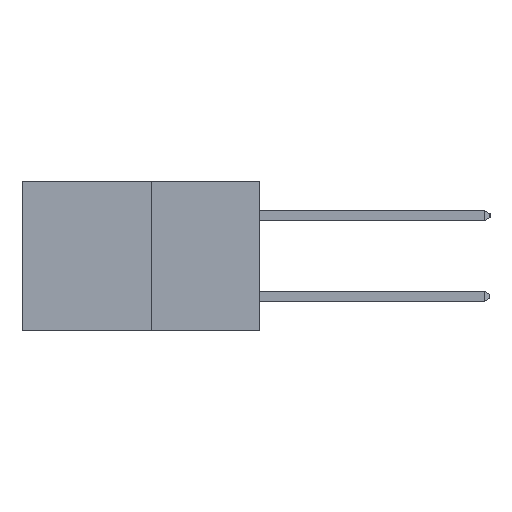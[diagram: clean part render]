
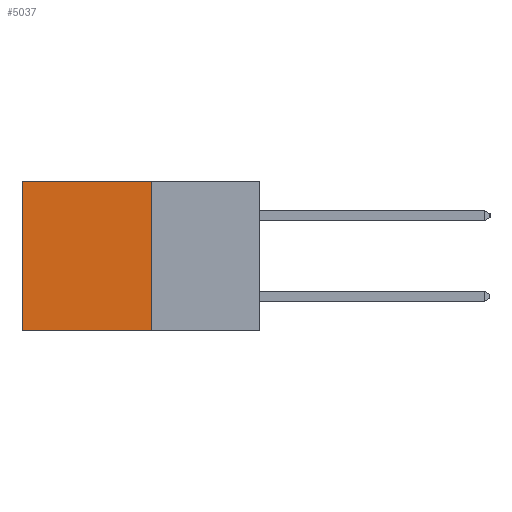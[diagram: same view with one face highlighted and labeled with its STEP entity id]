
A CAD part, left-side view. The second image highlights one B-rep face of the part: STEP entity #5037.
In plain terms, the highlighted planar face has unit normal (-1, 0, 0).
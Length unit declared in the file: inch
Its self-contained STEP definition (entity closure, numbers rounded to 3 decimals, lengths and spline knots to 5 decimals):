
#45 = CARTESIAN_POINT ( 'NONE',  ( 0.277, 0.59, -0.37 ) ) ;
#147 = CARTESIAN_POINT ( 'NONE',  ( 0.277, 0.27, 0. ) ) ;
#843 = VECTOR ( 'NONE', #1164, 39.37008 ) ;
#1095 = LINE ( 'NONE', #45, #843 ) ;
#1164 = DIRECTION ( 'NONE',  ( 0., 0., -1. ) ) ;
#1592 = LINE ( 'NONE', #4314, #1824 ) ;
#1748 = VECTOR ( 'NONE', #6209, 39.37008 ) ;
#1824 = VECTOR ( 'NONE', #4326, 39.37008 ) ;
#2028 = CARTESIAN_POINT ( 'NONE',  ( 0.277, 0.59, -0.37 ) ) ;
#2149 = VERTEX_POINT ( 'NONE', #147 ) ;
#2707 = VECTOR ( 'NONE', #7558, 39.37008 ) ;
#2893 = VERTEX_POINT ( 'NONE', #5431 ) ;
#3653 = ORIENTED_EDGE ( 'NONE', *, *, #7176, .T. ) ;
#3887 = LINE ( 'NONE', #6365, #1748 ) ;
#4292 = ORIENTED_EDGE ( 'NONE', *, *, #6542, .F. ) ;
#4314 = CARTESIAN_POINT ( 'NONE',  ( 0.277, 0.27, -0.37 ) ) ;
#4326 = DIRECTION ( 'NONE',  ( 0., 1., 0. ) ) ;
#4484 = ORIENTED_EDGE ( 'NONE', *, *, #9718, .F. ) ;
#4647 = EDGE_LOOP ( 'NONE', ( #3653, #4292, #4484, #5458 ) ) ;
#4763 = VERTEX_POINT ( 'NONE', #9887 ) ;
#5037 = ADVANCED_FACE ( 'NONE', ( #5525 ), #5830, .F. ) ;
#5375 = VERTEX_POINT ( 'NONE', #2028 ) ;
#5431 = CARTESIAN_POINT ( 'NONE',  ( 0.277, 0.27, -0.37 ) ) ;
#5458 = ORIENTED_EDGE ( 'NONE', *, *, #6231, .T. ) ;
#5525 = FACE_OUTER_BOUND ( 'NONE', #4647, .T. ) ;
#5694 = DIRECTION ( 'NONE',  ( 0., 0., -1. ) ) ;
#5706 = DIRECTION ( 'NONE',  ( 1., 0., 0. ) ) ;
#5830 = PLANE ( 'NONE',  #7362 ) ;
#5918 = CARTESIAN_POINT ( 'NONE',  ( 0.277, 0.27, -0.37 ) ) ;
#6209 = DIRECTION ( 'NONE',  ( 0., 0., -1. ) ) ;
#6231 = EDGE_CURVE ( 'NONE', #2149, #4763, #9211, .T. ) ;
#6365 = CARTESIAN_POINT ( 'NONE',  ( 0.277, 0.27, -0.37 ) ) ;
#6542 = EDGE_CURVE ( 'NONE', #2893, #5375, #1592, .T. ) ;
#7176 = EDGE_CURVE ( 'NONE', #4763, #5375, #1095, .T. ) ;
#7362 = AXIS2_PLACEMENT_3D ( 'NONE', #5918, #5706, #5694 ) ;
#7558 = DIRECTION ( 'NONE',  ( 0., 1., 0. ) ) ;
#7822 = CARTESIAN_POINT ( 'NONE',  ( 0.277, 0.27, 0. ) ) ;
#9211 = LINE ( 'NONE', #7822, #2707 ) ;
#9718 = EDGE_CURVE ( 'NONE', #2149, #2893, #3887, .T. ) ;
#9887 = CARTESIAN_POINT ( 'NONE',  ( 0.277, 0.59, 0. ) ) ;
